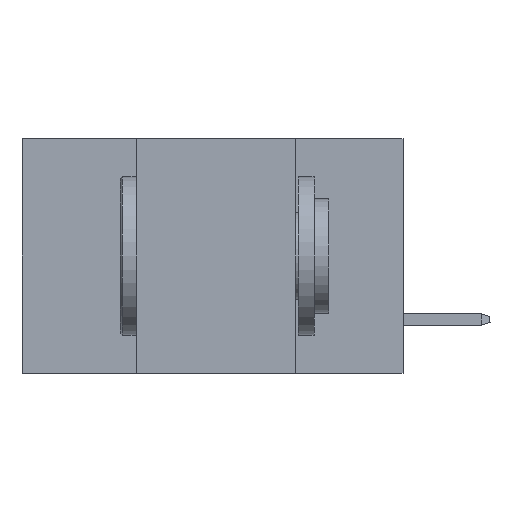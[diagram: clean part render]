
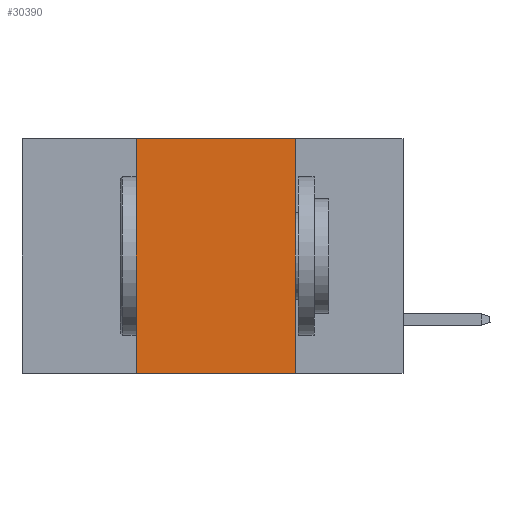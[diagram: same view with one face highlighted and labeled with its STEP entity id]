
A CAD part, left-side view. The second image highlights one B-rep face of the part: STEP entity #30390.
In plain terms, the highlighted planar face has unit normal (-1, 0, 0).
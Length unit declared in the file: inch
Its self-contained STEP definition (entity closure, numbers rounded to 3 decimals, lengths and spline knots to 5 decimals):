
#4668 = VECTOR ( 'NONE', #6098, 39.37008 ) ;
#6091 = ORIENTED_EDGE ( 'NONE', *, *, #19974, .F. ) ;
#6098 = DIRECTION ( 'NONE',  ( 0., 0., -1. ) ) ;
#8601 = DIRECTION ( 'NONE',  ( 0., 0., -1. ) ) ;
#8815 = DIRECTION ( 'NONE',  ( 1., 0., 0. ) ) ;
#8855 = AXIS2_PLACEMENT_3D ( 'NONE', #25137, #8815, #8601 ) ;
#8901 = DIRECTION ( 'NONE',  ( 0., -1., 0. ) ) ;
#9029 = PLANE ( 'NONE',  #8855 ) ;
#10581 = VECTOR ( 'NONE', #8901, 39.37008 ) ;
#10877 = CARTESIAN_POINT ( 'NONE',  ( 0., 0.17, -0.37 ) ) ;
#11321 = LINE ( 'NONE', #24173, #40598 ) ;
#11844 = VERTEX_POINT ( 'NONE', #16720 ) ;
#12838 = LINE ( 'NONE', #19585, #4668 ) ;
#14719 = VERTEX_POINT ( 'NONE', #10877 ) ;
#14947 = EDGE_CURVE ( 'NONE', #11844, #34030, #32621, .T. ) ;
#16720 = CARTESIAN_POINT ( 'NONE',  ( 0., 0.42, 0. ) ) ;
#18272 = DIRECTION ( 'NONE',  ( 0., -1., 0. ) ) ;
#19320 = VECTOR ( 'NONE', #42092, 39.37008 ) ;
#19585 = CARTESIAN_POINT ( 'NONE',  ( 0., 0.17, 0. ) ) ;
#19974 = EDGE_CURVE ( 'NONE', #34030, #14719, #12838, .T. ) ;
#22294 = FACE_OUTER_BOUND ( 'NONE', #40771, .T. ) ;
#22608 = EDGE_CURVE ( 'NONE', #35560, #11844, #32103, .T. ) ;
#24173 = CARTESIAN_POINT ( 'NONE',  ( 0., 0.6, -0.37 ) ) ;
#25137 = CARTESIAN_POINT ( 'NONE',  ( 0., 0.6, 0. ) ) ;
#25620 = CARTESIAN_POINT ( 'NONE',  ( 0., 0.42, -0.37 ) ) ;
#27713 = ORIENTED_EDGE ( 'NONE', *, *, #14947, .F. ) ;
#28825 = CARTESIAN_POINT ( 'NONE',  ( 0., 0.42, 0. ) ) ;
#30390 = ADVANCED_FACE ( 'NONE', ( #22294 ), #9029, .F. ) ;
#32103 = LINE ( 'NONE', #28825, #19320 ) ;
#32621 = LINE ( 'NONE', #38708, #10581 ) ;
#32719 = CARTESIAN_POINT ( 'NONE',  ( 0., 0.17, 0. ) ) ;
#33575 = ORIENTED_EDGE ( 'NONE', *, *, #22608, .F. ) ;
#34030 = VERTEX_POINT ( 'NONE', #32719 ) ;
#35560 = VERTEX_POINT ( 'NONE', #25620 ) ;
#38708 = CARTESIAN_POINT ( 'NONE',  ( 0., 0.6, 0. ) ) ;
#39357 = EDGE_CURVE ( 'NONE', #35560, #14719, #11321, .T. ) ;
#40598 = VECTOR ( 'NONE', #18272, 39.37008 ) ;
#40771 = EDGE_LOOP ( 'NONE', ( #6091, #27713, #33575, #41561 ) ) ;
#41561 = ORIENTED_EDGE ( 'NONE', *, *, #39357, .T. ) ;
#42092 = DIRECTION ( 'NONE',  ( 0., 0., 1. ) ) ;
